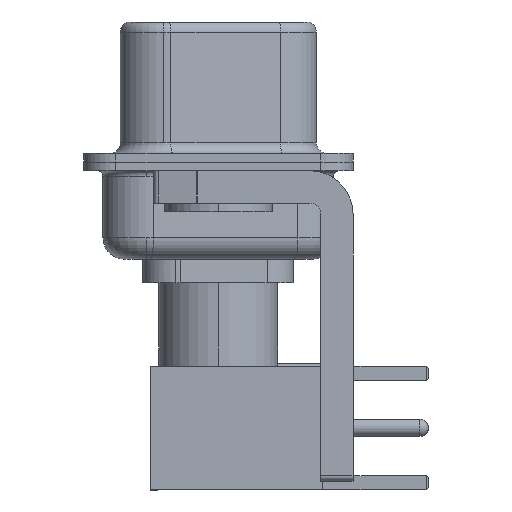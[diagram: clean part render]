
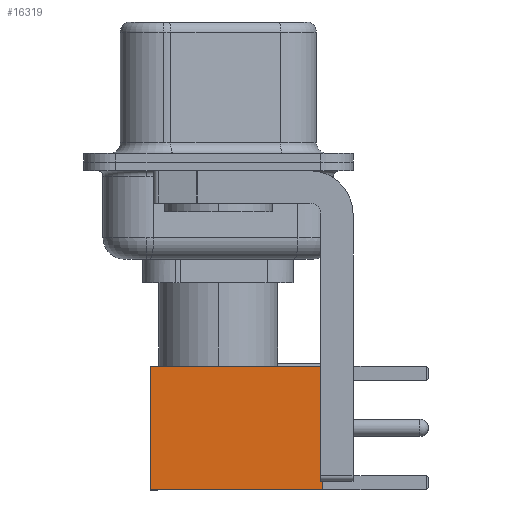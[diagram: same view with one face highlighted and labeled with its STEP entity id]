
A CAD part, left-side view. The second image highlights one B-rep face of the part: STEP entity #16319.
In plain terms, the highlighted face is planar.
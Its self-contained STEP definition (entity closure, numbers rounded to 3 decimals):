
#1903 = DIRECTION ( 'NONE',  ( 0., 0., 1. ) ) ;
#2691 = CARTESIAN_POINT ( 'NONE',  ( -2.875, 2.875, 0. ) ) ;
#4363 = DIRECTION ( 'NONE',  ( 0., 0., -1. ) ) ;
#4953 = VERTEX_POINT ( 'NONE', #2691 ) ;
#5439 = CARTESIAN_POINT ( 'NONE',  ( -2.875, 2.875, 0. ) ) ;
#5468 = CARTESIAN_POINT ( 'NONE',  ( -2.875, 2.875, 8. ) ) ;
#6149 = VECTOR ( 'NONE', #4363, 1000. ) ;
#6451 = CARTESIAN_POINT ( 'NONE',  ( 2.875, 2.875, 8. ) ) ;
#8470 = VERTEX_POINT ( 'NONE', #5468 ) ;
#8530 = EDGE_LOOP ( 'NONE', ( #20125, #17074, #19551, #24334 ) ) ;
#9224 = CARTESIAN_POINT ( 'NONE',  ( 0., 2.875, 8. ) ) ;
#9760 = LINE ( 'NONE', #9224, #15437 ) ;
#10332 = DIRECTION ( 'NONE',  ( 0., 1., 0. ) ) ;
#10351 = VECTOR ( 'NONE', #24610, 1000. ) ;
#11445 = EDGE_CURVE ( 'NONE', #17362, #19385, #16329, .T. ) ;
#12899 = LINE ( 'NONE', #22893, #10351 ) ;
#13711 = LINE ( 'NONE', #5439, #22568 ) ;
#14899 = CARTESIAN_POINT ( 'NONE',  ( 2.875, 2.875, 0. ) ) ;
#15437 = VECTOR ( 'NONE', #15669, 1000. ) ;
#15463 = PLANE ( 'NONE',  #21225 ) ;
#15669 = DIRECTION ( 'NONE',  ( -1., 0., 0. ) ) ;
#16319 = ADVANCED_FACE ( 'NONE', ( #25437 ), #15463, .T. ) ;
#16329 = LINE ( 'NONE', #24350, #6149 ) ;
#17015 = EDGE_CURVE ( 'NONE', #19385, #4953, #12899, .T. ) ;
#17074 = ORIENTED_EDGE ( 'NONE', *, *, #17015, .T. ) ;
#17362 = VERTEX_POINT ( 'NONE', #6451 ) ;
#18225 = CARTESIAN_POINT ( 'NONE',  ( 2.875, 2.875, 0. ) ) ;
#19385 = VERTEX_POINT ( 'NONE', #14899 ) ;
#19551 = ORIENTED_EDGE ( 'NONE', *, *, #19601, .F. ) ;
#19601 = EDGE_CURVE ( 'NONE', #8470, #4953, #13711, .T. ) ;
#20014 = EDGE_CURVE ( 'NONE', #17362, #8470, #9760, .T. ) ;
#20125 = ORIENTED_EDGE ( 'NONE', *, *, #11445, .T. ) ;
#21225 = AXIS2_PLACEMENT_3D ( 'NONE', #18225, #10332, #1903 ) ;
#21478 = DIRECTION ( 'NONE',  ( 0., 0., -1. ) ) ;
#22568 = VECTOR ( 'NONE', #21478, 1000. ) ;
#22893 = CARTESIAN_POINT ( 'NONE',  ( 0., 2.875, 0. ) ) ;
#24334 = ORIENTED_EDGE ( 'NONE', *, *, #20014, .F. ) ;
#24350 = CARTESIAN_POINT ( 'NONE',  ( 2.875, 2.875, 0. ) ) ;
#24610 = DIRECTION ( 'NONE',  ( -1., 0., 0. ) ) ;
#25437 = FACE_OUTER_BOUND ( 'NONE', #8530, .T. ) ;
